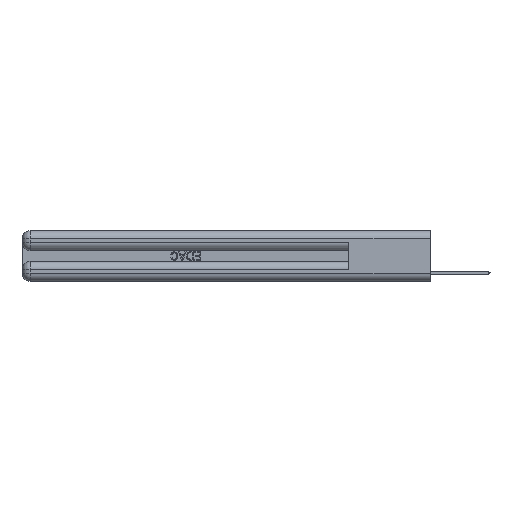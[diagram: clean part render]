
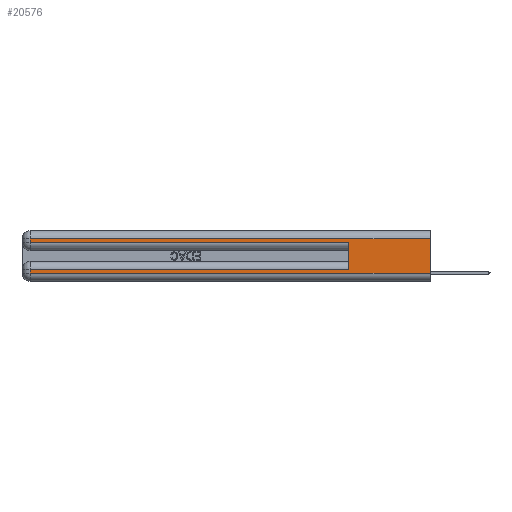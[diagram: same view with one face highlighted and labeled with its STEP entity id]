
A CAD part, left-side view. The second image highlights one B-rep face of the part: STEP entity #20576.
In plain terms, the highlighted planar face has unit normal (-1, 0, 0).
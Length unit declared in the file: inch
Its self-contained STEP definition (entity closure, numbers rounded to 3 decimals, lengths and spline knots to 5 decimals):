
#414 = ORIENTED_EDGE ( 'NONE', *, *, #31240, .T. ) ;
#681 = EDGE_CURVE ( 'NONE', #2723, #8916, #6843, .T. ) ;
#1400 = VECTOR ( 'NONE', #4686, 39.37008 ) ;
#2299 = DIRECTION ( 'NONE',  ( 0., -1., 0. ) ) ;
#2723 = VERTEX_POINT ( 'NONE', #6353 ) ;
#3210 = VERTEX_POINT ( 'NONE', #31108 ) ;
#3810 = LINE ( 'NONE', #26919, #17571 ) ;
#4053 = EDGE_CURVE ( 'NONE', #8916, #7951, #29008, .T. ) ;
#4686 = DIRECTION ( 'NONE',  ( 0., 0., -1. ) ) ;
#4730 = ORIENTED_EDGE ( 'NONE', *, *, #25873, .T. ) ;
#4906 = LINE ( 'NONE', #8962, #31020 ) ;
#5293 = LINE ( 'NONE', #6851, #24109 ) ;
#5546 = CARTESIAN_POINT ( 'NONE',  ( 0., 2.94, 0.06 ) ) ;
#6353 = CARTESIAN_POINT ( 'NONE',  ( 0., 0., 0.31 ) ) ;
#6813 = VECTOR ( 'NONE', #29069, 39.37008 ) ;
#6843 = LINE ( 'NONE', #24326, #17937 ) ;
#6851 = CARTESIAN_POINT ( 'NONE',  ( 0., 0.6, 0.145 ) ) ;
#7865 = VERTEX_POINT ( 'NONE', #11962 ) ;
#7951 = VERTEX_POINT ( 'NONE', #22237 ) ;
#8916 = VERTEX_POINT ( 'NONE', #11488 ) ;
#8962 = CARTESIAN_POINT ( 'NONE',  ( 0., 2.94, 0.37 ) ) ;
#10045 = DIRECTION ( 'NONE',  ( 0., 0., -1. ) ) ;
#10907 = EDGE_CURVE ( 'NONE', #21659, #15598, #4906, .T. ) ;
#11204 = ORIENTED_EDGE ( 'NONE', *, *, #19334, .T. ) ;
#11488 = CARTESIAN_POINT ( 'NONE',  ( 0., 2.94, 0.31 ) ) ;
#11962 = CARTESIAN_POINT ( 'NONE',  ( 0., 0.6, 0.085 ) ) ;
#12248 = DIRECTION ( 'NONE',  ( 0., -1., 0. ) ) ;
#12838 = DIRECTION ( 'NONE',  ( 1., 0., 0. ) ) ;
#14060 = LINE ( 'NONE', #26971, #6813 ) ;
#14109 = DIRECTION ( 'NONE',  ( 0., 0., 1. ) ) ;
#15598 = VERTEX_POINT ( 'NONE', #5546 ) ;
#15609 = VECTOR ( 'NONE', #2299, 39.37008 ) ;
#15679 = CARTESIAN_POINT ( 'NONE',  ( 0., 0., 0.37 ) ) ;
#16026 = LINE ( 'NONE', #16681, #15609 ) ;
#16426 = ORIENTED_EDGE ( 'NONE', *, *, #681, .T. ) ;
#16681 = CARTESIAN_POINT ( 'NONE',  ( 0., 0., 0.285 ) ) ;
#17571 = VECTOR ( 'NONE', #12248, 39.37008 ) ;
#17785 = EDGE_CURVE ( 'NONE', #2723, #25291, #27971, .T. ) ;
#17937 = VECTOR ( 'NONE', #26504, 39.37008 ) ;
#18161 = EDGE_CURVE ( 'NONE', #7865, #3210, #5293, .T. ) ;
#18474 = DIRECTION ( 'NONE',  ( 0., 0., -1. ) ) ;
#19190 = AXIS2_PLACEMENT_3D ( 'NONE', #27294, #12838, #10045 ) ;
#19334 = EDGE_CURVE ( 'NONE', #7865, #21659, #14060, .T. ) ;
#19534 = VECTOR ( 'NONE', #18474, 39.37008 ) ;
#20576 = ADVANCED_FACE ( 'NONE', ( #20629 ), #29675, .F. ) ;
#20629 = FACE_OUTER_BOUND ( 'NONE', #26738, .T. ) ;
#21179 = ORIENTED_EDGE ( 'NONE', *, *, #10907, .T. ) ;
#21659 = VERTEX_POINT ( 'NONE', #24406 ) ;
#22237 = CARTESIAN_POINT ( 'NONE',  ( 0., 2.94, 0.285 ) ) ;
#24109 = VECTOR ( 'NONE', #14109, 39.37008 ) ;
#24326 = CARTESIAN_POINT ( 'NONE',  ( 0., 0., 0.31 ) ) ;
#24330 = ORIENTED_EDGE ( 'NONE', *, *, #18161, .F. ) ;
#24406 = CARTESIAN_POINT ( 'NONE',  ( 0., 2.94, 0.085 ) ) ;
#25291 = VERTEX_POINT ( 'NONE', #28803 ) ;
#25873 = EDGE_CURVE ( 'NONE', #7951, #3210, #16026, .T. ) ;
#26396 = ORIENTED_EDGE ( 'NONE', *, *, #4053, .T. ) ;
#26504 = DIRECTION ( 'NONE',  ( 0., 1., 0. ) ) ;
#26738 = EDGE_LOOP ( 'NONE', ( #29114, #16426, #26396, #4730, #24330, #11204, #21179, #414 ) ) ;
#26833 = CARTESIAN_POINT ( 'NONE',  ( 0., 2.94, 0.37 ) ) ;
#26919 = CARTESIAN_POINT ( 'NONE',  ( 0., 0., 0.06 ) ) ;
#26971 = CARTESIAN_POINT ( 'NONE',  ( 0., 0., 0.085 ) ) ;
#27294 = CARTESIAN_POINT ( 'NONE',  ( 0., 0., 0.37 ) ) ;
#27971 = LINE ( 'NONE', #15679, #19534 ) ;
#28453 = DIRECTION ( 'NONE',  ( 0., 0., -1. ) ) ;
#28803 = CARTESIAN_POINT ( 'NONE',  ( 0., 0., 0.06 ) ) ;
#29008 = LINE ( 'NONE', #26833, #1400 ) ;
#29069 = DIRECTION ( 'NONE',  ( 0., 1., 0. ) ) ;
#29114 = ORIENTED_EDGE ( 'NONE', *, *, #17785, .F. ) ;
#29675 = PLANE ( 'NONE',  #19190 ) ;
#31020 = VECTOR ( 'NONE', #28453, 39.37008 ) ;
#31108 = CARTESIAN_POINT ( 'NONE',  ( 0., 0.6, 0.285 ) ) ;
#31240 = EDGE_CURVE ( 'NONE', #15598, #25291, #3810, .T. ) ;
